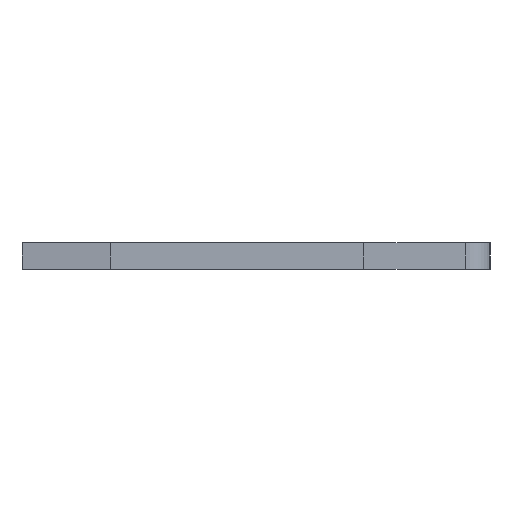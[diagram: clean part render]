
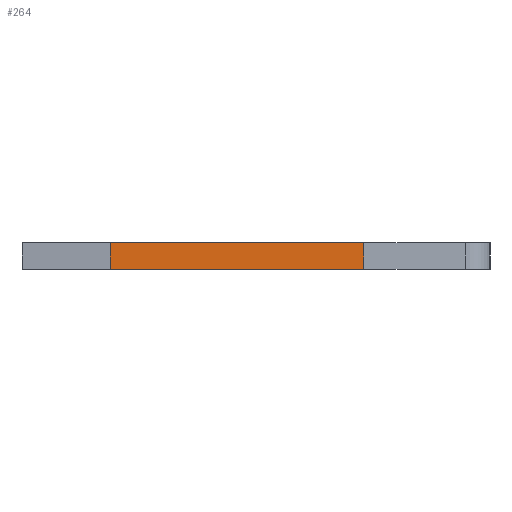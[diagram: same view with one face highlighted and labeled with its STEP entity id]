
A CAD part, left-side view. The second image highlights one B-rep face of the part: STEP entity #264.
In plain terms, the highlighted face is planar.
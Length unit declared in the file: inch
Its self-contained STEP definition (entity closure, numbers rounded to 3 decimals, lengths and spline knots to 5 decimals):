
#24 = CARTESIAN_POINT ( 'NONE',  ( -0.013, 0.146, -0.0575 ) ) ;
#111 = CARTESIAN_POINT ( 'NONE',  ( 0.013, 0.146, -0.0575 ) ) ;
#142 = VERTEX_POINT ( 'NONE', #232 ) ;
#203 = ORIENTED_EDGE ( 'NONE', *, *, #243, .T. ) ;
#220 = VERTEX_POINT ( 'NONE', #971 ) ;
#232 = CARTESIAN_POINT ( 'NONE',  ( 0.013, -0.099, -0.0575 ) ) ;
#243 = EDGE_CURVE ( 'NONE', #142, #1000, #1366, .T. ) ;
#264 = ADVANCED_FACE ( 'NONE', ( #816 ), #1125, .F. ) ;
#275 = EDGE_CURVE ( 'NONE', #940, #220, #645, .T. ) ;
#294 = VECTOR ( 'NONE', #1550, 39.37008 ) ;
#363 = CARTESIAN_POINT ( 'NONE',  ( 0.013, 0.146, -0.0575 ) ) ;
#496 = DIRECTION ( 'NONE',  ( 0., 1., 0. ) ) ;
#546 = VECTOR ( 'NONE', #496, 39.37008 ) ;
#600 = EDGE_CURVE ( 'NONE', #142, #940, #1097, .T. ) ;
#645 = LINE ( 'NONE', #363, #939 ) ;
#682 = LINE ( 'NONE', #24, #294 ) ;
#686 = VECTOR ( 'NONE', #868, 39.37008 ) ;
#692 = ORIENTED_EDGE ( 'NONE', *, *, #600, .F. ) ;
#697 = CARTESIAN_POINT ( 'NONE',  ( 0.013, 0.146, -0.0575 ) ) ;
#816 = FACE_OUTER_BOUND ( 'NONE', #1122, .T. ) ;
#853 = DIRECTION ( 'NONE',  ( 1., 0., 0. ) ) ;
#868 = DIRECTION ( 'NONE',  ( -1., 0., 0. ) ) ;
#915 = ORIENTED_EDGE ( 'NONE', *, *, #275, .F. ) ;
#939 = VECTOR ( 'NONE', #1482, 39.37008 ) ;
#940 = VERTEX_POINT ( 'NONE', #697 ) ;
#971 = CARTESIAN_POINT ( 'NONE',  ( -0.013, 0.146, -0.0575 ) ) ;
#978 = ORIENTED_EDGE ( 'NONE', *, *, #1512, .T. ) ;
#987 = DIRECTION ( 'NONE',  ( 0., 0., 1. ) ) ;
#1000 = VERTEX_POINT ( 'NONE', #1345 ) ;
#1097 = LINE ( 'NONE', #1529, #546 ) ;
#1122 = EDGE_LOOP ( 'NONE', ( #978, #915, #692, #203 ) ) ;
#1125 = PLANE ( 'NONE',  #1585 ) ;
#1252 = CARTESIAN_POINT ( 'NONE',  ( 0.013, -0.099, -0.0575 ) ) ;
#1345 = CARTESIAN_POINT ( 'NONE',  ( -0.013, -0.099, -0.0575 ) ) ;
#1366 = LINE ( 'NONE', #1252, #686 ) ;
#1482 = DIRECTION ( 'NONE',  ( -1., 0., 0. ) ) ;
#1512 = EDGE_CURVE ( 'NONE', #1000, #220, #682, .T. ) ;
#1529 = CARTESIAN_POINT ( 'NONE',  ( 0.013, 0.146, -0.0575 ) ) ;
#1550 = DIRECTION ( 'NONE',  ( 0., 1., 0. ) ) ;
#1585 = AXIS2_PLACEMENT_3D ( 'NONE', #111, #987, #853 ) ;
